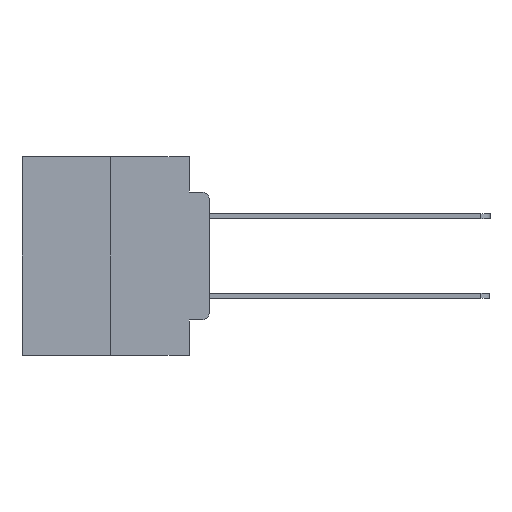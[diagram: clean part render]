
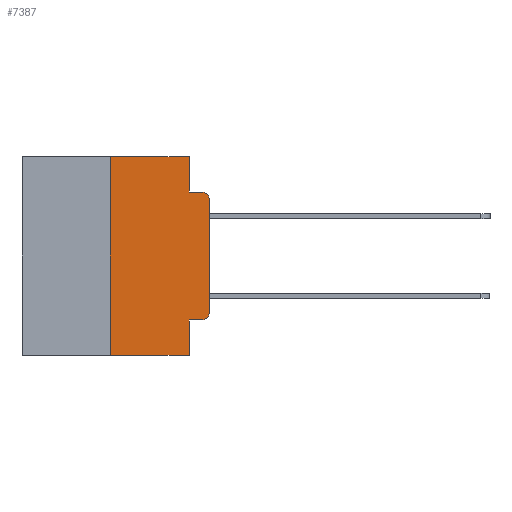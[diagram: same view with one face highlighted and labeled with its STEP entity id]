
A CAD part, left-side view. The second image highlights one B-rep face of the part: STEP entity #7387.
In plain terms, the highlighted planar face has unit normal (-1, 0, 0).
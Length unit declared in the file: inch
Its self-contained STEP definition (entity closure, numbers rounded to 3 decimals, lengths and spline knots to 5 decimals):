
#760 = CARTESIAN_POINT ( 'NONE',  ( 0., 0.051, 0. ) ) ;
#781 = ORIENTED_EDGE ( 'NONE', *, *, #24250, .T. ) ;
#1475 = ORIENTED_EDGE ( 'NONE', *, *, #10539, .F. ) ;
#1525 = CARTESIAN_POINT ( 'NONE',  ( 0., 0.051, -0.0885 ) ) ;
#1727 = CARTESIAN_POINT ( 'NONE',  ( 0., 0.25, 0. ) ) ;
#2496 = VERTEX_POINT ( 'NONE', #25948 ) ;
#2707 = DIRECTION ( 'NONE',  ( 0., 0., 1. ) ) ;
#3503 = ORIENTED_EDGE ( 'NONE', *, *, #9665, .T. ) ;
#3696 = DIRECTION ( 'NONE',  ( 0., -1., 0. ) ) ;
#3726 = DIRECTION ( 'NONE',  ( 0., -1., 0. ) ) ;
#3840 = VECTOR ( 'NONE', #24164, 39.37008 ) ;
#4071 = AXIS2_PLACEMENT_3D ( 'NONE', #19981, #7515, #21972 ) ;
#4218 = LINE ( 'NONE', #24085, #9279 ) ;
#4285 = DIRECTION ( 'NONE',  ( 1., 0., 0. ) ) ;
#4870 = VECTOR ( 'NONE', #2707, 39.37008 ) ;
#5061 = LINE ( 'NONE', #23412, #14350 ) ;
#5325 = CARTESIAN_POINT ( 'NONE',  ( 0., 0., -0.3915 ) ) ;
#5360 = EDGE_CURVE ( 'NONE', #10963, #9835, #9627, .T. ) ;
#5665 = CARTESIAN_POINT ( 'NONE',  ( 0., 0.051, 0. ) ) ;
#5987 = CARTESIAN_POINT ( 'NONE',  ( 0., 0.473, -0.5 ) ) ;
#7387 = ADVANCED_FACE ( 'NONE', ( #9849 ), #22903, .F. ) ;
#7515 = DIRECTION ( 'NONE',  ( -1., 0., 0. ) ) ;
#7769 = VERTEX_POINT ( 'NONE', #11894 ) ;
#7895 = VERTEX_POINT ( 'NONE', #1727 ) ;
#8643 = VERTEX_POINT ( 'NONE', #23109 ) ;
#8816 = CARTESIAN_POINT ( 'NONE',  ( 0., 0.051, -0.5 ) ) ;
#9279 = VECTOR ( 'NONE', #26087, 39.37008 ) ;
#9560 = LINE ( 'NONE', #18167, #3840 ) ;
#9627 = CIRCLE ( 'NONE', #18981, 0.02 ) ;
#9635 = VECTOR ( 'NONE', #3696, 39.37008 ) ;
#9665 = EDGE_CURVE ( 'NONE', #8643, #10963, #5061, .T. ) ;
#9835 = VERTEX_POINT ( 'NONE', #5325 ) ;
#9849 = FACE_OUTER_BOUND ( 'NONE', #16677, .T. ) ;
#10539 = EDGE_CURVE ( 'NONE', #14075, #13146, #15542, .T. ) ;
#10607 = VECTOR ( 'NONE', #3726, 39.37008 ) ;
#10905 = DIRECTION ( 'NONE',  ( 0., 0., -1. ) ) ;
#10963 = VERTEX_POINT ( 'NONE', #17462 ) ;
#11894 = CARTESIAN_POINT ( 'NONE',  ( 0., 0.25, -0.5 ) ) ;
#12145 = ORIENTED_EDGE ( 'NONE', *, *, #16184, .F. ) ;
#12699 = CIRCLE ( 'NONE', #4071, 0.02 ) ;
#13146 = VERTEX_POINT ( 'NONE', #16727 ) ;
#13284 = DIRECTION ( 'NONE',  ( 0., -1., 0. ) ) ;
#13451 = CARTESIAN_POINT ( 'NONE',  ( 0., 0.02, -0.0885 ) ) ;
#13489 = ORIENTED_EDGE ( 'NONE', *, *, #21867, .F. ) ;
#14075 = VERTEX_POINT ( 'NONE', #760 ) ;
#14350 = VECTOR ( 'NONE', #13284, 39.37008 ) ;
#14864 = VECTOR ( 'NONE', #26189, 39.37008 ) ;
#15423 = DIRECTION ( 'NONE',  ( -1., 0., 0. ) ) ;
#15476 = CARTESIAN_POINT ( 'NONE',  ( 0., 0.25, 0. ) ) ;
#15490 = ORIENTED_EDGE ( 'NONE', *, *, #5360, .T. ) ;
#15542 = LINE ( 'NONE', #5665, #14864 ) ;
#15999 = CARTESIAN_POINT ( 'NONE',  ( 0., 0.02, -0.3915 ) ) ;
#16184 = EDGE_CURVE ( 'NONE', #13146, #19598, #20614, .T. ) ;
#16456 = VECTOR ( 'NONE', #22140, 39.37008 ) ;
#16677 = EDGE_LOOP ( 'NONE', ( #17113, #781, #12145, #1475, #23648, #13489, #24291, #19619, #3503, #15490 ) ) ;
#16727 = CARTESIAN_POINT ( 'NONE',  ( 0., 0.051, -0.0885 ) ) ;
#17113 = ORIENTED_EDGE ( 'NONE', *, *, #26926, .T. ) ;
#17462 = CARTESIAN_POINT ( 'NONE',  ( 0., 0.02, -0.4115 ) ) ;
#18167 = CARTESIAN_POINT ( 'NONE',  ( 0., 0.051, 0. ) ) ;
#18250 = CARTESIAN_POINT ( 'NONE',  ( 0., 0.473, 0. ) ) ;
#18835 = VERTEX_POINT ( 'NONE', #8816 ) ;
#18981 = AXIS2_PLACEMENT_3D ( 'NONE', #15999, #15423, #10905 ) ;
#19006 = DIRECTION ( 'NONE',  ( 0., 0., -1. ) ) ;
#19598 = VERTEX_POINT ( 'NONE', #13451 ) ;
#19619 = ORIENTED_EDGE ( 'NONE', *, *, #22063, .F. ) ;
#19981 = CARTESIAN_POINT ( 'NONE',  ( 0., 0.02, -0.1085 ) ) ;
#20614 = LINE ( 'NONE', #1525, #9635 ) ;
#21867 = EDGE_CURVE ( 'NONE', #7769, #7895, #26807, .T. ) ;
#21972 = DIRECTION ( 'NONE',  ( 0., 0., -1. ) ) ;
#22063 = EDGE_CURVE ( 'NONE', #8643, #18835, #9560, .T. ) ;
#22088 = EDGE_CURVE ( 'NONE', #7895, #14075, #25213, .T. ) ;
#22140 = DIRECTION ( 'NONE',  ( 0., -1., 0. ) ) ;
#22656 = AXIS2_PLACEMENT_3D ( 'NONE', #26944, #4285, #19006 ) ;
#22903 = PLANE ( 'NONE',  #22656 ) ;
#23109 = CARTESIAN_POINT ( 'NONE',  ( 0., 0.051, -0.4115 ) ) ;
#23412 = CARTESIAN_POINT ( 'NONE',  ( 0., 0.051, -0.4115 ) ) ;
#23648 = ORIENTED_EDGE ( 'NONE', *, *, #22088, .F. ) ;
#24085 = CARTESIAN_POINT ( 'NONE',  ( 0., 0., 0. ) ) ;
#24164 = DIRECTION ( 'NONE',  ( 0., 0., -1. ) ) ;
#24250 = EDGE_CURVE ( 'NONE', #2496, #19598, #12699, .T. ) ;
#24291 = ORIENTED_EDGE ( 'NONE', *, *, #26426, .T. ) ;
#25213 = LINE ( 'NONE', #18250, #16456 ) ;
#25948 = CARTESIAN_POINT ( 'NONE',  ( 0., 0., -0.1085 ) ) ;
#26087 = DIRECTION ( 'NONE',  ( 0., 0., 1. ) ) ;
#26189 = DIRECTION ( 'NONE',  ( 0., 0., -1. ) ) ;
#26426 = EDGE_CURVE ( 'NONE', #7769, #18835, #26865, .T. ) ;
#26807 = LINE ( 'NONE', #15476, #4870 ) ;
#26865 = LINE ( 'NONE', #5987, #10607 ) ;
#26926 = EDGE_CURVE ( 'NONE', #9835, #2496, #4218, .T. ) ;
#26944 = CARTESIAN_POINT ( 'NONE',  ( 0., 0.473, 0. ) ) ;
